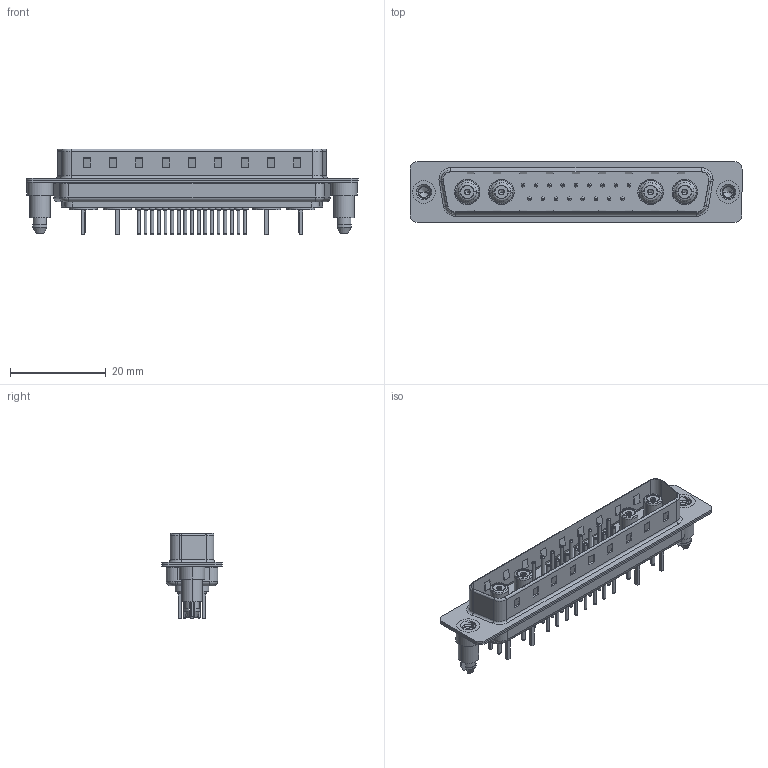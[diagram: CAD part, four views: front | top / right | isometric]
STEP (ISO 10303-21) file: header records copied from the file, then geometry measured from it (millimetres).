
FILE_DESCRIPTION (( 'STEP AP203' ), '1' );
FILE_NAME ('627-21W4224-7T5.STEP', '2019-05-30T11:04:50', ( '' ), ( '' ), 'SwSTEP 2.0', 'SolidWorks 2016', '' );
FILE_SCHEMA (( 'CONFIG_CONTROL_DESIGN' ));
Length unit declared in the file: millimetre
Products named in the file (13): Locking Collar; Socket_Str; 627Combo Housing_21W4; Co-Ax Jack Assy_S; 627Combo Shell Rear_37 Contacts; 627Combo Contact Row 1_24; 627Combo Shell Front_37 Contacts; 627Combo Contact Row 2_24; 627Combo Threaded Boardlock_5; 627-21W4224-7T5; Co-Ax Jack_Straight PC Tail; Insulator Socket; Insulator Socket 2
Assembly tree (31 placements, depth 3):
  627-21W4224-7T5
    627Combo Housing_21W4
    627Combo Shell Rear_37 Contacts
    627Combo Shell Front_37 Contacts
    627Combo Threaded Boardlock_5  x2
    Co-Ax Jack Assy_S  x4
      Co-Ax Jack_Straight PC Tail
      Insulator Socket
      Insulator Socket 2
      Locking Collar
      Socket_Str
    627Combo Contact Row 1_24  x9
    627Combo Contact Row 2_24  x8
Bounding box: 69.3 x 12.6 x 17.9 mm (x, y, z)
Volume: 3987.1 mm3; surface area: 11093.9 mm2
Topology: 42 solids, 42 shells, 1535 faces, 3443 edges, 2124 vertices
Faces by surface type: cylinder 599, plane 526, torus 338, cone 50, bspline 14, sphere 8
Entity records: 24943 total; most frequent: CARTESIAN_POINT 5458, DIRECTION 3912, ORIENTED_EDGE 3474, EDGE_CURVE 1737, AXIS2_PLACEMENT_3D 1505, VERTEX_POINT 1105, LINE 902, VECTOR 902
